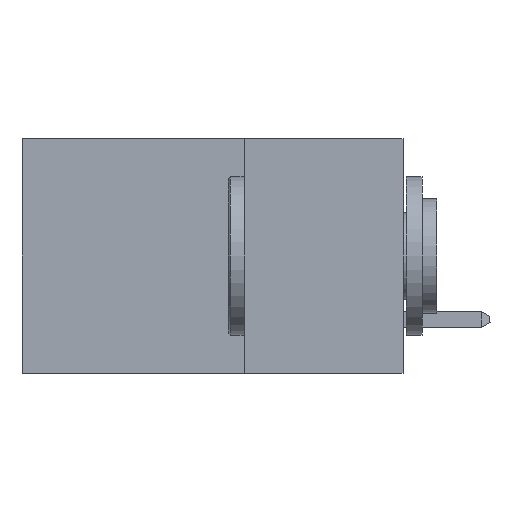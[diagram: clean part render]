
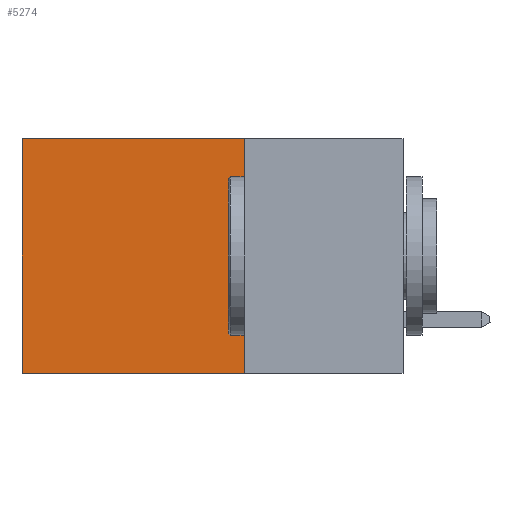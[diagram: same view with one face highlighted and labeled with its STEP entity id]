
A CAD part, left-side view. The second image highlights one B-rep face of the part: STEP entity #5274.
In plain terms, the highlighted planar face has unit normal (-1, 0, 0).
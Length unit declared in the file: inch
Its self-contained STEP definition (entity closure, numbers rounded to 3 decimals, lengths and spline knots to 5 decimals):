
#998 = LINE ( 'NONE', #5934, #18329 ) ;
#1111 = CARTESIAN_POINT ( 'NONE',  ( 0.2875, 0.25, -0.37 ) ) ;
#1888 = DIRECTION ( 'NONE',  ( 0., 0., -1. ) ) ;
#2431 = CARTESIAN_POINT ( 'NONE',  ( 0.2875, 0.6, 0. ) ) ;
#2818 = ORIENTED_EDGE ( 'NONE', *, *, #9644, .T. ) ;
#3110 = LINE ( 'NONE', #2431, #23001 ) ;
#3899 = DIRECTION ( 'NONE',  ( 0., 1., 0. ) ) ;
#5274 = ADVANCED_FACE ( 'NONE', ( #8895 ), #8180, .F. ) ;
#5934 = CARTESIAN_POINT ( 'NONE',  ( 0.2875, 0.25, 0. ) ) ;
#6126 = CARTESIAN_POINT ( 'NONE',  ( 0.2875, 0.25, 0. ) ) ;
#7553 = VERTEX_POINT ( 'NONE', #23391 ) ;
#8090 = DIRECTION ( 'NONE',  ( 0., 0., -1. ) ) ;
#8106 = ORIENTED_EDGE ( 'NONE', *, *, #12956, .F. ) ;
#8180 = PLANE ( 'NONE',  #18896 ) ;
#8895 = FACE_OUTER_BOUND ( 'NONE', #9602, .T. ) ;
#9602 = EDGE_LOOP ( 'NONE', ( #19870, #8106, #15306, #2818 ) ) ;
#9644 = EDGE_CURVE ( 'NONE', #23205, #23246, #998, .T. ) ;
#11003 = LINE ( 'NONE', #12822, #11282 ) ;
#11282 = VECTOR ( 'NONE', #12672, 39.37008 ) ;
#11711 = EDGE_CURVE ( 'NONE', #23246, #7553, #3110, .T. ) ;
#11759 = VECTOR ( 'NONE', #1888, 39.37008 ) ;
#12226 = CARTESIAN_POINT ( 'NONE',  ( 0.2875, 0.25, 0. ) ) ;
#12672 = DIRECTION ( 'NONE',  ( 0., 1., 0. ) ) ;
#12787 = VERTEX_POINT ( 'NONE', #1111 ) ;
#12822 = CARTESIAN_POINT ( 'NONE',  ( 0.2875, 0.25, -0.37 ) ) ;
#12956 = EDGE_CURVE ( 'NONE', #12787, #7553, #11003, .T. ) ;
#13914 = DIRECTION ( 'NONE',  ( 0., 0., -1. ) ) ;
#15306 = ORIENTED_EDGE ( 'NONE', *, *, #22079, .F. ) ;
#17990 = CARTESIAN_POINT ( 'NONE',  ( 0.2875, 0.6, 0. ) ) ;
#18329 = VECTOR ( 'NONE', #3899, 39.37008 ) ;
#18852 = CARTESIAN_POINT ( 'NONE',  ( 0.2875, 0.25, 0. ) ) ;
#18896 = AXIS2_PLACEMENT_3D ( 'NONE', #6126, #19239, #8090 ) ;
#19239 = DIRECTION ( 'NONE',  ( 1., 0., 0. ) ) ;
#19870 = ORIENTED_EDGE ( 'NONE', *, *, #11711, .T. ) ;
#20858 = LINE ( 'NONE', #18852, #11759 ) ;
#22079 = EDGE_CURVE ( 'NONE', #23205, #12787, #20858, .T. ) ;
#23001 = VECTOR ( 'NONE', #13914, 39.37008 ) ;
#23205 = VERTEX_POINT ( 'NONE', #12226 ) ;
#23246 = VERTEX_POINT ( 'NONE', #17990 ) ;
#23391 = CARTESIAN_POINT ( 'NONE',  ( 0.2875, 0.6, -0.37 ) ) ;
